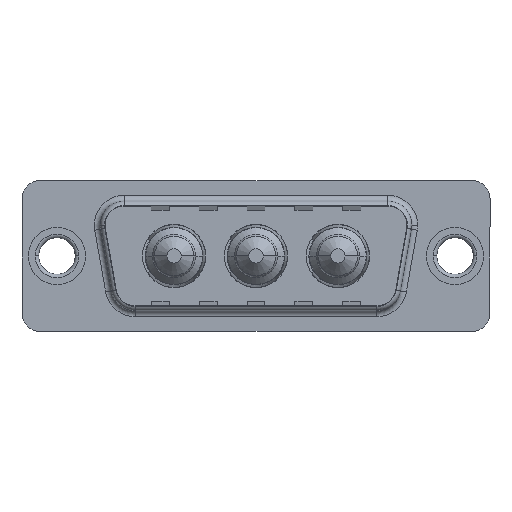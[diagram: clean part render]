
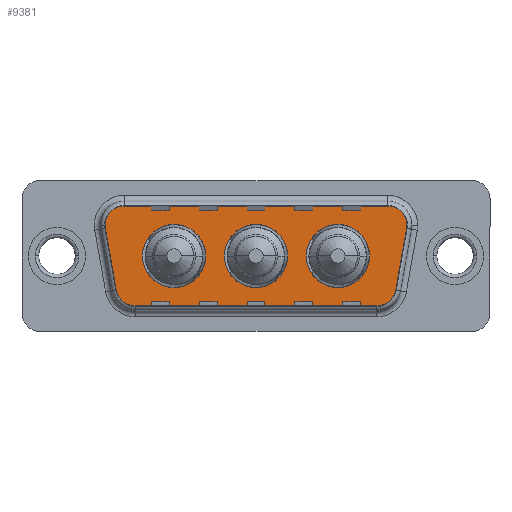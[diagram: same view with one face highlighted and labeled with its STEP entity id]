
A CAD part, top view. The second image highlights one B-rep face of the part: STEP entity #9381.
In plain terms, the highlighted planar face has unit normal (0, 0, 1).
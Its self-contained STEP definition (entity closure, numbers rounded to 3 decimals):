
#155 = AXIS2_PLACEMENT_3D ( 'NONE', #3912, #1640, #7110 ) ;
#270 = VERTEX_POINT ( 'NONE', #3811 ) ;
#382 = LINE ( 'NONE', #10017, #7310 ) ;
#406 = ORIENTED_EDGE ( 'NONE', *, *, #4249, .T. ) ;
#567 = CARTESIAN_POINT ( 'NONE',  ( 19.3, 0., 0. ) ) ;
#831 = DIRECTION ( 'NONE',  ( 0., 0., 1. ) ) ;
#845 = CARTESIAN_POINT ( 'NONE',  ( 23.5, 0., 0. ) ) ;
#897 = VECTOR ( 'NONE', #3929, 1000. ) ;
#968 = CIRCLE ( 'NONE', #9367, 2.65 ) ;
#1037 = VERTEX_POINT ( 'NONE', #8434 ) ;
#1046 = CARTESIAN_POINT ( 'NONE',  ( 3.441, 2.553, 0. ) ) ;
#1079 = VERTEX_POINT ( 'NONE', #1046 ) ;
#1354 = EDGE_CURVE ( 'NONE', #5584, #7665, #968, .T. ) ;
#1377 = FACE_BOUND ( 'NONE', #9149, .T. ) ;
#1393 = CARTESIAN_POINT ( 'NONE',  ( 12.45, 0., 0. ) ) ;
#1476 = CARTESIAN_POINT ( 'NONE',  ( 6.434, -2.9, 0. ) ) ;
#1568 = AXIS2_PLACEMENT_3D ( 'NONE', #4243, #10299, #5120 ) ;
#1640 = DIRECTION ( 'NONE',  ( 0., 0., 1. ) ) ;
#1690 = CARTESIAN_POINT ( 'NONE',  ( 4.464, -3.247, 0. ) ) ;
#1707 = DIRECTION ( 'NONE',  ( 1., 0., 0. ) ) ;
#1941 = LINE ( 'NONE', #6903, #4250 ) ;
#2011 = DIRECTION ( 'NONE',  ( 0., 0., 1. ) ) ;
#2105 = ORIENTED_EDGE ( 'NONE', *, *, #7958, .F. ) ;
#2137 = DIRECTION ( 'NONE',  ( 0., 0., 1. ) ) ;
#2199 = CIRCLE ( 'NONE', #9487, 2.65 ) ;
#2264 = CARTESIAN_POINT ( 'NONE',  ( 3.441, 2.553, 0. ) ) ;
#2276 = EDGE_CURVE ( 'NONE', #4004, #270, #9486, .T. ) ;
#2347 = DIRECTION ( 'NONE',  ( -1., 0., 0. ) ) ;
#2405 = EDGE_LOOP ( 'NONE', ( #9218, #5962, #406, #9999, #10569, #7879, #7012, #8851, #3129 ) ) ;
#2471 = CARTESIAN_POINT ( 'NONE',  ( 26.866, -4.9, 0. ) ) ;
#2479 = VECTOR ( 'NONE', #8312, 1000. ) ;
#2507 = CARTESIAN_POINT ( 'NONE',  ( 26.15, 0., 0. ) ) ;
#2531 = VERTEX_POINT ( 'NONE', #567 ) ;
#2571 = EDGE_CURVE ( 'NONE', #270, #4735, #382, .T. ) ;
#2572 = AXIS2_PLACEMENT_3D ( 'NONE', #3536, #9602, #4430 ) ;
#2644 = CIRCLE ( 'NONE', #8790, 2.65 ) ;
#2848 = CARTESIAN_POINT ( 'NONE',  ( 16.65, 0., 0. ) ) ;
#2854 = CARTESIAN_POINT ( 'NONE',  ( 7.15, 0., 0. ) ) ;
#2885 = CIRCLE ( 'NONE', #7215, 2.65 ) ;
#2996 = CIRCLE ( 'NONE', #3055, 2.65 ) ;
#3055 = AXIS2_PLACEMENT_3D ( 'NONE', #845, #6920, #1707 ) ;
#3129 = ORIENTED_EDGE ( 'NONE', *, *, #11227, .T. ) ;
#3223 = CARTESIAN_POINT ( 'NONE',  ( 14., 0., 0. ) ) ;
#3244 = VERTEX_POINT ( 'NONE', #6116 ) ;
#3255 = CARTESIAN_POINT ( 'NONE',  ( 29.889, 2.9, 0. ) ) ;
#3378 = ORIENTED_EDGE ( 'NONE', *, *, #1354, .F. ) ;
#3411 = CARTESIAN_POINT ( 'NONE',  ( 5.411, 4.9, 0. ) ) ;
#3480 = CARTESIAN_POINT ( 'NONE',  ( 26.866, -2.9, 0. ) ) ;
#3494 = CARTESIAN_POINT ( 'NONE',  ( 27.889, 4.9, 0. ) ) ;
#3536 = CARTESIAN_POINT ( 'NONE',  ( 23.5, 0., 0. ) ) ;
#3597 = ORIENTED_EDGE ( 'NONE', *, *, #5901, .F. ) ;
#3673 = FACE_BOUND ( 'NONE', #7079, .T. ) ;
#3681 = ORIENTED_EDGE ( 'NONE', *, *, #8085, .F. ) ;
#3727 = DIRECTION ( 'NONE',  ( 1., 0., 0. ) ) ;
#3811 = CARTESIAN_POINT ( 'NONE',  ( 28.836, -3.247, 0. ) ) ;
#3899 = DIRECTION ( 'NONE',  ( 1., 0., 0. ) ) ;
#3912 = CARTESIAN_POINT ( 'NONE',  ( 5.411, 2.9, 0. ) ) ;
#3929 = DIRECTION ( 'NONE',  ( -1., 0., 0. ) ) ;
#4004 = VERTEX_POINT ( 'NONE', #2471 ) ;
#4243 = CARTESIAN_POINT ( 'NONE',  ( 27.889, 2.9, 0. ) ) ;
#4249 = EDGE_CURVE ( 'NONE', #4735, #11101, #4562, .T. ) ;
#4250 = VECTOR ( 'NONE', #4316, 1000. ) ;
#4316 = DIRECTION ( 'NONE',  ( 1., 0., 0. ) ) ;
#4388 = DIRECTION ( 'NONE',  ( -1., 0., 0. ) ) ;
#4430 = DIRECTION ( 'NONE',  ( 1., 0., 0. ) ) ;
#4562 = CIRCLE ( 'NONE', #7517, 2. ) ;
#4568 = CARTESIAN_POINT ( 'NONE',  ( 9.8, 0., 0. ) ) ;
#4670 = EDGE_CURVE ( 'NONE', #7938, #9411, #10100, .T. ) ;
#4706 = ORIENTED_EDGE ( 'NONE', *, *, #8792, .F. ) ;
#4735 = VERTEX_POINT ( 'NONE', #5674 ) ;
#5032 = CARTESIAN_POINT ( 'NONE',  ( 16.65, 0., 0. ) ) ;
#5038 = EDGE_CURVE ( 'NONE', #9411, #1079, #6043, .T. ) ;
#5120 = DIRECTION ( 'NONE',  ( -1., 0., 0. ) ) ;
#5220 = DIRECTION ( 'NONE',  ( 0., 0., 1. ) ) ;
#5584 = VERTEX_POINT ( 'NONE', #2854 ) ;
#5628 = EDGE_LOOP ( 'NONE', ( #6001, #3681 ) ) ;
#5674 = CARTESIAN_POINT ( 'NONE',  ( 29.859, 2.553, 0. ) ) ;
#5711 = FACE_BOUND ( 'NONE', #5628, .T. ) ;
#5899 = DIRECTION ( 'NONE',  ( 1., 0., 0. ) ) ;
#5901 = EDGE_CURVE ( 'NONE', #7665, #5584, #2644, .T. ) ;
#5962 = ORIENTED_EDGE ( 'NONE', *, *, #2571, .T. ) ;
#6001 = ORIENTED_EDGE ( 'NONE', *, *, #11122, .F. ) ;
#6043 = CIRCLE ( 'NONE', #155, 2. ) ;
#6097 = CARTESIAN_POINT ( 'NONE',  ( 27.889, 2.9, 0. ) ) ;
#6116 = CARTESIAN_POINT ( 'NONE',  ( 20.85, 0., 0. ) ) ;
#6193 = DIRECTION ( 'NONE',  ( 0.174, 0.985, 0. ) ) ;
#6277 = LINE ( 'NONE', #2264, #2479 ) ;
#6623 = DIRECTION ( 'NONE',  ( 1., 0., 0. ) ) ;
#6789 = AXIS2_PLACEMENT_3D ( 'NONE', #3480, #2011, #3899 ) ;
#6900 = DIRECTION ( 'NONE',  ( 1., 0., 0. ) ) ;
#6903 = CARTESIAN_POINT ( 'NONE',  ( 6.434, -4.9, 0. ) ) ;
#6920 = DIRECTION ( 'NONE',  ( 0., 0., 1. ) ) ;
#7012 = ORIENTED_EDGE ( 'NONE', *, *, #7145, .T. ) ;
#7079 = EDGE_LOOP ( 'NONE', ( #3597, #3378 ) ) ;
#7110 = DIRECTION ( 'NONE',  ( 1., 0., 0. ) ) ;
#7145 = EDGE_CURVE ( 'NONE', #1079, #11222, #6277, .T. ) ;
#7177 = EDGE_CURVE ( 'NONE', #11222, #1037, #10336, .T. ) ;
#7215 = AXIS2_PLACEMENT_3D ( 'NONE', #2848, #8905, #3727 ) ;
#7249 = VERTEX_POINT ( 'NONE', #2507 ) ;
#7310 = VECTOR ( 'NONE', #6193, 1000. ) ;
#7517 = AXIS2_PLACEMENT_3D ( 'NONE', #6097, #5220, #4388 ) ;
#7539 = DIRECTION ( 'NONE',  ( 0., 0., 1. ) ) ;
#7665 = VERTEX_POINT ( 'NONE', #1393 ) ;
#7879 = ORIENTED_EDGE ( 'NONE', *, *, #5038, .T. ) ;
#7938 = VERTEX_POINT ( 'NONE', #3494 ) ;
#7958 = EDGE_CURVE ( 'NONE', #3244, #7249, #11162, .T. ) ;
#8003 = FACE_OUTER_BOUND ( 'NONE', #2405, .T. ) ;
#8085 = EDGE_CURVE ( 'NONE', #11086, #2531, #2885, .T. ) ;
#8312 = DIRECTION ( 'NONE',  ( 0.174, -0.985, 0. ) ) ;
#8434 = CARTESIAN_POINT ( 'NONE',  ( 6.434, -4.9, 0. ) ) ;
#8790 = AXIS2_PLACEMENT_3D ( 'NONE', #4568, #9209, #11178 ) ;
#8792 = EDGE_CURVE ( 'NONE', #7249, #3244, #2996, .T. ) ;
#8851 = ORIENTED_EDGE ( 'NONE', *, *, #7177, .T. ) ;
#8868 = AXIS2_PLACEMENT_3D ( 'NONE', #1476, #7539, #2347 ) ;
#8905 = DIRECTION ( 'NONE',  ( 0., 0., 1. ) ) ;
#9144 = CARTESIAN_POINT ( 'NONE',  ( 5.411, 4.9, 0. ) ) ;
#9149 = EDGE_LOOP ( 'NONE', ( #4706, #2105 ) ) ;
#9209 = DIRECTION ( 'NONE',  ( 0., 0., 1. ) ) ;
#9218 = ORIENTED_EDGE ( 'NONE', *, *, #2276, .T. ) ;
#9367 = AXIS2_PLACEMENT_3D ( 'NONE', #10224, #2137, #6623 ) ;
#9381 = ADVANCED_FACE ( 'NONE', ( #5711, #1377, #3673, #8003 ), #11189, .T. ) ;
#9411 = VERTEX_POINT ( 'NONE', #3411 ) ;
#9486 = CIRCLE ( 'NONE', #6789, 2. ) ;
#9487 = AXIS2_PLACEMENT_3D ( 'NONE', #5032, #11087, #5899 ) ;
#9602 = DIRECTION ( 'NONE',  ( 0., 0., 1. ) ) ;
#9999 = ORIENTED_EDGE ( 'NONE', *, *, #10688, .T. ) ;
#10017 = CARTESIAN_POINT ( 'NONE',  ( 29.859, 2.553, 0. ) ) ;
#10100 = LINE ( 'NONE', #9144, #897 ) ;
#10198 = AXIS2_PLACEMENT_3D ( 'NONE', #10326, #831, #6900 ) ;
#10224 = CARTESIAN_POINT ( 'NONE',  ( 9.8, 0., 0. ) ) ;
#10299 = DIRECTION ( 'NONE',  ( 0., 0., 1. ) ) ;
#10326 = CARTESIAN_POINT ( 'NONE',  ( 26.866, -2.9, 0. ) ) ;
#10336 = CIRCLE ( 'NONE', #8868, 2. ) ;
#10446 = CIRCLE ( 'NONE', #1568, 2. ) ;
#10569 = ORIENTED_EDGE ( 'NONE', *, *, #4670, .T. ) ;
#10688 = EDGE_CURVE ( 'NONE', #11101, #7938, #10446, .T. ) ;
#11086 = VERTEX_POINT ( 'NONE', #3223 ) ;
#11087 = DIRECTION ( 'NONE',  ( 0., 0., 1. ) ) ;
#11101 = VERTEX_POINT ( 'NONE', #3255 ) ;
#11122 = EDGE_CURVE ( 'NONE', #2531, #11086, #2199, .T. ) ;
#11162 = CIRCLE ( 'NONE', #2572, 2.65 ) ;
#11178 = DIRECTION ( 'NONE',  ( 1., 0., 0. ) ) ;
#11189 = PLANE ( 'NONE',  #10198 ) ;
#11222 = VERTEX_POINT ( 'NONE', #1690 ) ;
#11227 = EDGE_CURVE ( 'NONE', #1037, #4004, #1941, .T. ) ;
